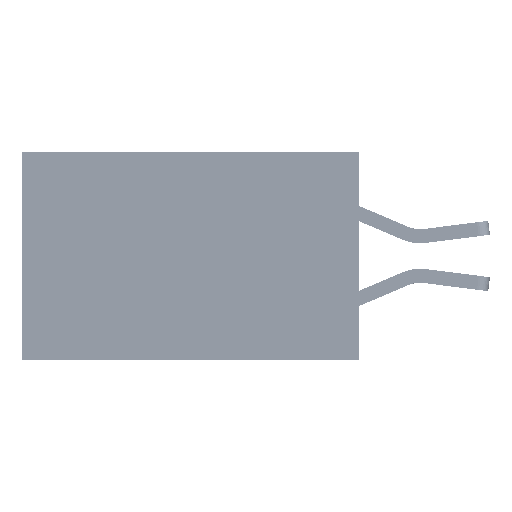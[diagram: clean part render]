
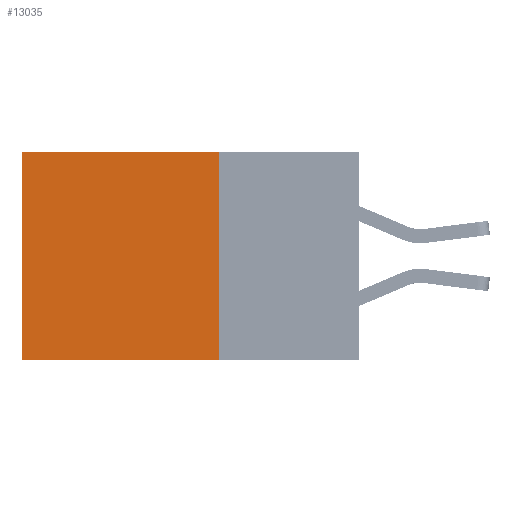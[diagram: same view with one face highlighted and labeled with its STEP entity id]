
A CAD part, left-side view. The second image highlights one B-rep face of the part: STEP entity #13035.
In plain terms, the highlighted planar face has unit normal (-1, 0, 0).
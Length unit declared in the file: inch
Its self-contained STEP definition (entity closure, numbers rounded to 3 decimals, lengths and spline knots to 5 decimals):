
#1312 = CARTESIAN_POINT ( 'NONE',  ( 0.2875, 0.25, -0.37 ) ) ;
#1695 = DIRECTION ( 'NONE',  ( 0., 0., -1. ) ) ;
#1836 = EDGE_LOOP ( 'NONE', ( #23361, #13502, #35948, #38627 ) ) ;
#3931 = VERTEX_POINT ( 'NONE', #33341 ) ;
#5022 = DIRECTION ( 'NONE',  ( 0., 1., 0. ) ) ;
#5523 = VECTOR ( 'NONE', #5022, 39.37008 ) ;
#6382 = VECTOR ( 'NONE', #31164, 39.37008 ) ;
#6935 = CARTESIAN_POINT ( 'NONE',  ( 0.2875, 0.25, -0.37 ) ) ;
#8269 = VERTEX_POINT ( 'NONE', #26714 ) ;
#9363 = VECTOR ( 'NONE', #23682, 39.37008 ) ;
#9453 = CARTESIAN_POINT ( 'NONE',  ( 0.2875, 0.6, 0. ) ) ;
#10431 = VERTEX_POINT ( 'NONE', #1312 ) ;
#10687 = LINE ( 'NONE', #6935, #6382 ) ;
#12272 = CARTESIAN_POINT ( 'NONE',  ( 0.2875, 0.25, 0. ) ) ;
#13035 = ADVANCED_FACE ( 'NONE', ( #34654 ), #37598, .F. ) ;
#13476 = DIRECTION ( 'NONE',  ( 1., 0., 0. ) ) ;
#13502 = ORIENTED_EDGE ( 'NONE', *, *, #37325, .F. ) ;
#13764 = VECTOR ( 'NONE', #1695, 39.37008 ) ;
#17291 = AXIS2_PLACEMENT_3D ( 'NONE', #37750, #13476, #34531 ) ;
#18256 = EDGE_CURVE ( 'NONE', #32019, #8269, #31007, .T. ) ;
#23361 = ORIENTED_EDGE ( 'NONE', *, *, #39833, .T. ) ;
#23682 = DIRECTION ( 'NONE',  ( 0., 0., -1. ) ) ;
#26714 = CARTESIAN_POINT ( 'NONE',  ( 0.2875, 0.6, 0. ) ) ;
#26791 = EDGE_CURVE ( 'NONE', #32019, #10431, #32216, .T. ) ;
#31007 = LINE ( 'NONE', #35091, #5523 ) ;
#31164 = DIRECTION ( 'NONE',  ( 0., 1., 0. ) ) ;
#32019 = VERTEX_POINT ( 'NONE', #32153 ) ;
#32153 = CARTESIAN_POINT ( 'NONE',  ( 0.2875, 0.25, 0. ) ) ;
#32216 = LINE ( 'NONE', #12272, #13764 ) ;
#33341 = CARTESIAN_POINT ( 'NONE',  ( 0.2875, 0.6, -0.37 ) ) ;
#34531 = DIRECTION ( 'NONE',  ( 0., 0., -1. ) ) ;
#34654 = FACE_OUTER_BOUND ( 'NONE', #1836, .T. ) ;
#35091 = CARTESIAN_POINT ( 'NONE',  ( 0.2875, 0.25, 0. ) ) ;
#35948 = ORIENTED_EDGE ( 'NONE', *, *, #26791, .F. ) ;
#37030 = LINE ( 'NONE', #9453, #9363 ) ;
#37325 = EDGE_CURVE ( 'NONE', #10431, #3931, #10687, .T. ) ;
#37598 = PLANE ( 'NONE',  #17291 ) ;
#37750 = CARTESIAN_POINT ( 'NONE',  ( 0.2875, 0.25, 0. ) ) ;
#38627 = ORIENTED_EDGE ( 'NONE', *, *, #18256, .T. ) ;
#39833 = EDGE_CURVE ( 'NONE', #8269, #3931, #37030, .T. ) ;
